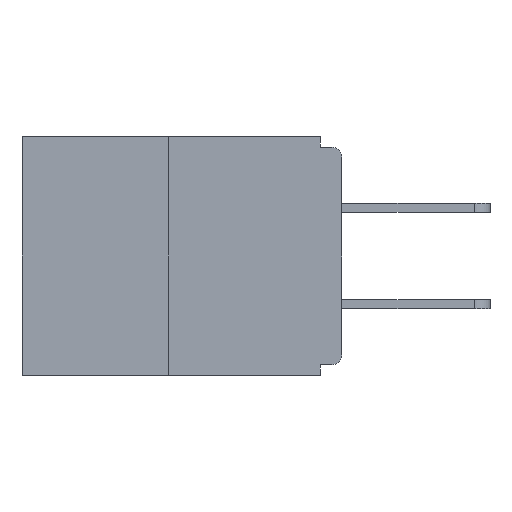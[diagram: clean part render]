
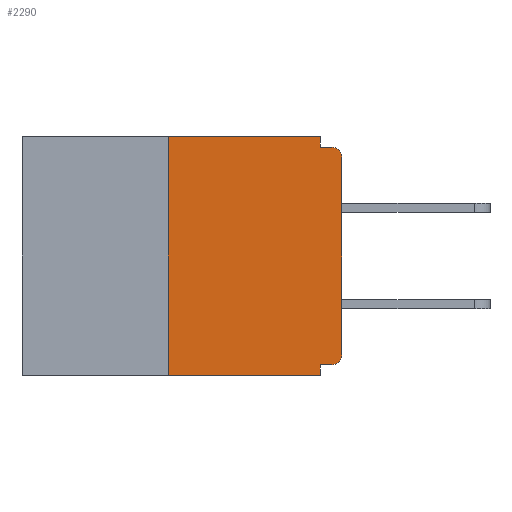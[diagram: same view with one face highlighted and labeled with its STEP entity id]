
A CAD part, left-side view. The second image highlights one B-rep face of the part: STEP entity #2290.
In plain terms, the highlighted planar face has unit normal (-1, 0, 0).
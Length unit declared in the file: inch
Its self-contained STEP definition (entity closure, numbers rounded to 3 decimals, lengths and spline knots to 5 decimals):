
#126 = FACE_OUTER_BOUND ( 'NONE', #12820, .T. ) ;
#473 = EDGE_CURVE ( 'NONE', #10051, #11852, #13551, .T. ) ;
#793 = DIRECTION ( 'NONE',  ( 1., 0., 0. ) ) ;
#1133 = VERTEX_POINT ( 'NONE', #5216 ) ;
#1209 = EDGE_CURVE ( 'NONE', #10051, #14153, #5574, .T. ) ;
#1236 = PLANE ( 'NONE',  #9583 ) ;
#1282 = CARTESIAN_POINT ( 'NONE',  ( 0., 0.25, 0. ) ) ;
#1801 = ORIENTED_EDGE ( 'NONE', *, *, #10593, .T. ) ;
#1904 = CARTESIAN_POINT ( 'NONE',  ( 0., 0.46, -0.343 ) ) ;
#2114 = VECTOR ( 'NONE', #14802, 39.37008 ) ;
#2214 = LINE ( 'NONE', #7936, #4306 ) ;
#2290 = ADVANCED_FACE ( 'NONE', ( #126 ), #1236, .F. ) ;
#2380 = ORIENTED_EDGE ( 'NONE', *, *, #10505, .F. ) ;
#2784 = DIRECTION ( 'NONE',  ( 0., 0., 1. ) ) ;
#3135 = CARTESIAN_POINT ( 'NONE',  ( 0., 0., -0.313 ) ) ;
#3483 = DIRECTION ( 'NONE',  ( 0., 0., -1. ) ) ;
#3730 = CARTESIAN_POINT ( 'NONE',  ( 0., 0.031, 0. ) ) ;
#4306 = VECTOR ( 'NONE', #3483, 39.37008 ) ;
#4337 = CARTESIAN_POINT ( 'NONE',  ( 0., 0., -0.328 ) ) ;
#4637 = CARTESIAN_POINT ( 'NONE',  ( 0., 0.25, 0. ) ) ;
#5216 = CARTESIAN_POINT ( 'NONE',  ( 0., 0.015, -0.015 ) ) ;
#5574 = CIRCLE ( 'NONE', #16407, 0.015 ) ;
#5652 = VERTEX_POINT ( 'NONE', #6377 ) ;
#5971 = EDGE_CURVE ( 'NONE', #11852, #9259, #2214, .T. ) ;
#6160 = DIRECTION ( 'NONE',  ( -1., 0., 0. ) ) ;
#6377 = CARTESIAN_POINT ( 'NONE',  ( 0., 0.031, -0.015 ) ) ;
#6539 = EDGE_CURVE ( 'NONE', #5652, #1133, #17167, .T. ) ;
#6577 = ORIENTED_EDGE ( 'NONE', *, *, #7497, .F. ) ;
#6626 = CIRCLE ( 'NONE', #9178, 0.015 ) ;
#6669 = CARTESIAN_POINT ( 'NONE',  ( 0., 0., -0.03 ) ) ;
#6772 = CARTESIAN_POINT ( 'NONE',  ( 0., 0.25, -0.343 ) ) ;
#6824 = DIRECTION ( 'NONE',  ( -1., 0., 0. ) ) ;
#6921 = EDGE_CURVE ( 'NONE', #14777, #9259, #16181, .T. ) ;
#7197 = CARTESIAN_POINT ( 'NONE',  ( 0., 0.46, 0. ) ) ;
#7405 = LINE ( 'NONE', #13842, #10471 ) ;
#7497 = EDGE_CURVE ( 'NONE', #14777, #17425, #14792, .T. ) ;
#7666 = DIRECTION ( 'NONE',  ( 0., 0., -1. ) ) ;
#7781 = VECTOR ( 'NONE', #18352, 39.37008 ) ;
#7797 = LINE ( 'NONE', #3730, #14803 ) ;
#7936 = CARTESIAN_POINT ( 'NONE',  ( 0., 0.031, -0.343 ) ) ;
#9178 = AXIS2_PLACEMENT_3D ( 'NONE', #12112, #6160, #7666 ) ;
#9259 = VERTEX_POINT ( 'NONE', #16581 ) ;
#9405 = CARTESIAN_POINT ( 'NONE',  ( 0., 0.015, -0.328 ) ) ;
#9434 = VECTOR ( 'NONE', #2784, 39.37008 ) ;
#9583 = AXIS2_PLACEMENT_3D ( 'NONE', #7197, #793, #17673 ) ;
#9954 = ORIENTED_EDGE ( 'NONE', *, *, #473, .F. ) ;
#10051 = VERTEX_POINT ( 'NONE', #9405 ) ;
#10471 = VECTOR ( 'NONE', #10670, 39.37008 ) ;
#10505 = EDGE_CURVE ( 'NONE', #17425, #18070, #10931, .T. ) ;
#10577 = ORIENTED_EDGE ( 'NONE', *, *, #1209, .T. ) ;
#10593 = EDGE_CURVE ( 'NONE', #14153, #15197, #7405, .T. ) ;
#10670 = DIRECTION ( 'NONE',  ( 0., 0., 1. ) ) ;
#10931 = LINE ( 'NONE', #19422, #19331 ) ;
#11433 = ORIENTED_EDGE ( 'NONE', *, *, #17871, .T. ) ;
#11852 = VERTEX_POINT ( 'NONE', #13468 ) ;
#12112 = CARTESIAN_POINT ( 'NONE',  ( 0., 0.015, -0.03 ) ) ;
#12621 = ORIENTED_EDGE ( 'NONE', *, *, #6921, .T. ) ;
#12789 = DIRECTION ( 'NONE',  ( 0., 0., -1. ) ) ;
#12820 = EDGE_LOOP ( 'NONE', ( #2380, #6577, #12621, #16123, #9954, #10577, #1801, #11433, #18894, #17927 ) ) ;
#12824 = EDGE_CURVE ( 'NONE', #18070, #5652, #7797, .T. ) ;
#13468 = CARTESIAN_POINT ( 'NONE',  ( 0., 0.031, -0.328 ) ) ;
#13551 = LINE ( 'NONE', #4337, #2114 ) ;
#13842 = CARTESIAN_POINT ( 'NONE',  ( 0., 0., 0. ) ) ;
#14153 = VERTEX_POINT ( 'NONE', #3135 ) ;
#14414 = DIRECTION ( 'NONE',  ( 0., 0., -1. ) ) ;
#14777 = VERTEX_POINT ( 'NONE', #6772 ) ;
#14792 = LINE ( 'NONE', #1282, #9434 ) ;
#14802 = DIRECTION ( 'NONE',  ( 0., 1., 0. ) ) ;
#14803 = VECTOR ( 'NONE', #12789, 39.37008 ) ;
#14837 = DIRECTION ( 'NONE',  ( 0., -1., 0. ) ) ;
#14927 = DIRECTION ( 'NONE',  ( 0., -1., 0. ) ) ;
#15197 = VERTEX_POINT ( 'NONE', #6669 ) ;
#15587 = CARTESIAN_POINT ( 'NONE',  ( 0., 0., -0.015 ) ) ;
#16123 = ORIENTED_EDGE ( 'NONE', *, *, #5971, .F. ) ;
#16181 = LINE ( 'NONE', #1904, #7781 ) ;
#16407 = AXIS2_PLACEMENT_3D ( 'NONE', #18848, #6824, #14414 ) ;
#16581 = CARTESIAN_POINT ( 'NONE',  ( 0., 0.031, -0.343 ) ) ;
#17167 = LINE ( 'NONE', #15587, #19019 ) ;
#17425 = VERTEX_POINT ( 'NONE', #4637 ) ;
#17673 = DIRECTION ( 'NONE',  ( 0., 0., -1. ) ) ;
#17871 = EDGE_CURVE ( 'NONE', #15197, #1133, #6626, .T. ) ;
#17927 = ORIENTED_EDGE ( 'NONE', *, *, #12824, .F. ) ;
#18070 = VERTEX_POINT ( 'NONE', #18250 ) ;
#18250 = CARTESIAN_POINT ( 'NONE',  ( 0., 0.031, 0. ) ) ;
#18352 = DIRECTION ( 'NONE',  ( 0., -1., 0. ) ) ;
#18848 = CARTESIAN_POINT ( 'NONE',  ( 0., 0.015, -0.313 ) ) ;
#18894 = ORIENTED_EDGE ( 'NONE', *, *, #6539, .F. ) ;
#19019 = VECTOR ( 'NONE', #14927, 39.37008 ) ;
#19331 = VECTOR ( 'NONE', #14837, 39.37008 ) ;
#19422 = CARTESIAN_POINT ( 'NONE',  ( 0., 0.46, 0. ) ) ;
